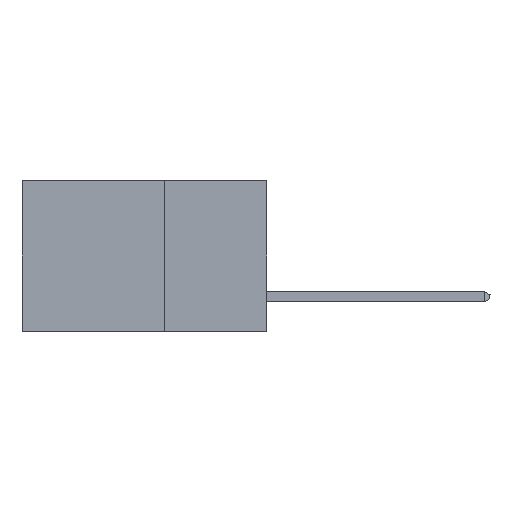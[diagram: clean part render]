
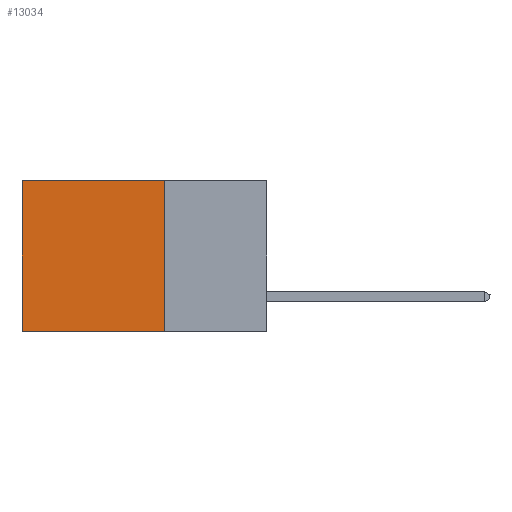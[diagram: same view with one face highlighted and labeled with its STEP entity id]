
A CAD part, left-side view. The second image highlights one B-rep face of the part: STEP entity #13034.
In plain terms, the highlighted planar face has unit normal (-1, 0, 0).
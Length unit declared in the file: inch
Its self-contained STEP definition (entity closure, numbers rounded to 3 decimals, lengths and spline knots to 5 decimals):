
#488 = AXIS2_PLACEMENT_3D ( 'NONE', #5019, #21787, #12422 ) ;
#1040 = EDGE_CURVE ( 'NONE', #7957, #6986, #17597, .T. ) ;
#3705 = ORIENTED_EDGE ( 'NONE', *, *, #1040, .F. ) ;
#3947 = CARTESIAN_POINT ( 'NONE',  ( 0.2875, 0.25, -0.37 ) ) ;
#3977 = EDGE_CURVE ( 'NONE', #10641, #6986, #9055, .T. ) ;
#4956 = VERTEX_POINT ( 'NONE', #5911 ) ;
#5019 = CARTESIAN_POINT ( 'NONE',  ( 0.2875, 0.25, 0. ) ) ;
#5888 = EDGE_CURVE ( 'NONE', #4956, #7957, #14972, .T. ) ;
#5911 = CARTESIAN_POINT ( 'NONE',  ( 0.2875, 0.25, 0. ) ) ;
#6986 = VERTEX_POINT ( 'NONE', #14604 ) ;
#7957 = VERTEX_POINT ( 'NONE', #3947 ) ;
#8022 = VECTOR ( 'NONE', #13941, 39.37008 ) ;
#8052 = CARTESIAN_POINT ( 'NONE',  ( 0.2875, 0.25, 0. ) ) ;
#9055 = LINE ( 'NONE', #20491, #23565 ) ;
#9402 = DIRECTION ( 'NONE',  ( 0., 0., -1. ) ) ;
#9568 = CARTESIAN_POINT ( 'NONE',  ( 0.2875, 0.25, 0. ) ) ;
#10641 = VERTEX_POINT ( 'NONE', #23744 ) ;
#10926 = VECTOR ( 'NONE', #20871, 39.37008 ) ;
#12344 = EDGE_CURVE ( 'NONE', #4956, #10641, #13551, .T. ) ;
#12422 = DIRECTION ( 'NONE',  ( 0., 0., -1. ) ) ;
#12723 = ORIENTED_EDGE ( 'NONE', *, *, #5888, .F. ) ;
#13034 = ADVANCED_FACE ( 'NONE', ( #23750 ), #14356, .F. ) ;
#13551 = LINE ( 'NONE', #9568, #10926 ) ;
#13941 = DIRECTION ( 'NONE',  ( 0., 1., 0. ) ) ;
#14356 = PLANE ( 'NONE',  #488 ) ;
#14604 = CARTESIAN_POINT ( 'NONE',  ( 0.2875, 0.6, -0.37 ) ) ;
#14972 = LINE ( 'NONE', #8052, #21535 ) ;
#15034 = ORIENTED_EDGE ( 'NONE', *, *, #12344, .T. ) ;
#17597 = LINE ( 'NONE', #23203, #8022 ) ;
#17628 = EDGE_LOOP ( 'NONE', ( #20723, #3705, #12723, #15034 ) ) ;
#18411 = DIRECTION ( 'NONE',  ( 0., 0., -1. ) ) ;
#20491 = CARTESIAN_POINT ( 'NONE',  ( 0.2875, 0.6, 0. ) ) ;
#20723 = ORIENTED_EDGE ( 'NONE', *, *, #3977, .T. ) ;
#20871 = DIRECTION ( 'NONE',  ( 0., 1., 0. ) ) ;
#21535 = VECTOR ( 'NONE', #9402, 39.37008 ) ;
#21787 = DIRECTION ( 'NONE',  ( 1., 0., 0. ) ) ;
#23203 = CARTESIAN_POINT ( 'NONE',  ( 0.2875, 0.25, -0.37 ) ) ;
#23565 = VECTOR ( 'NONE', #18411, 39.37008 ) ;
#23744 = CARTESIAN_POINT ( 'NONE',  ( 0.2875, 0.6, 0. ) ) ;
#23750 = FACE_OUTER_BOUND ( 'NONE', #17628, .T. ) ;
